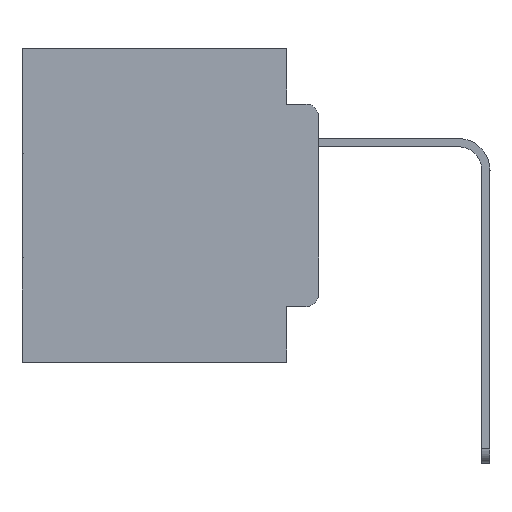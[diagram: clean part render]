
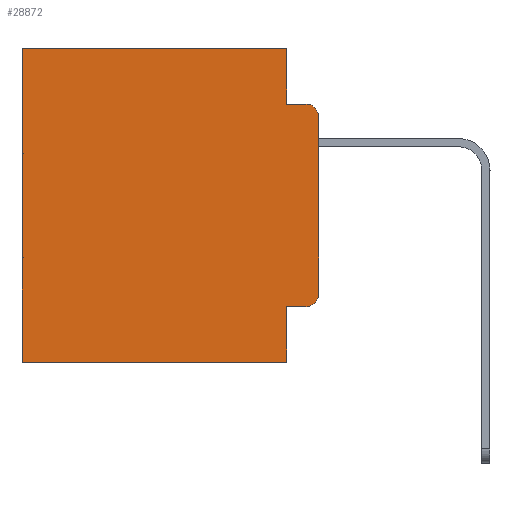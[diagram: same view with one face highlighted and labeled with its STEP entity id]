
A CAD part, left-side view. The second image highlights one B-rep face of the part: STEP entity #28872.
In plain terms, the highlighted planar face has unit normal (-1, 0, 0).
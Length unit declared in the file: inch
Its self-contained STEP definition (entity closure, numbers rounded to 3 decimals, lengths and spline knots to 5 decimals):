
#457 = AXIS2_PLACEMENT_3D ( 'NONE', #6395, #11030, #6303 ) ;
#1258 = VECTOR ( 'NONE', #29152, 39.37008 ) ;
#1271 = VERTEX_POINT ( 'NONE', #6291 ) ;
#1674 = LINE ( 'NONE', #18268, #20343 ) ;
#1702 = LINE ( 'NONE', #28573, #14700 ) ;
#1807 = EDGE_CURVE ( 'NONE', #15006, #8651, #1702, .T. ) ;
#2079 = EDGE_CURVE ( 'NONE', #19711, #15006, #1674, .T. ) ;
#3271 = VECTOR ( 'NONE', #3747, 39.37008 ) ;
#3747 = DIRECTION ( 'NONE',  ( 0., 1., 0. ) ) ;
#3829 = DIRECTION ( 'NONE',  ( 0., 0., -1. ) ) ;
#3906 = CARTESIAN_POINT ( 'NONE',  ( 0.298, 0.473, -0.5 ) ) ;
#4085 = VECTOR ( 'NONE', #28516, 39.37008 ) ;
#4306 = EDGE_CURVE ( 'NONE', #5901, #17204, #14968, .T. ) ;
#4488 = ORIENTED_EDGE ( 'NONE', *, *, #25899, .T. ) ;
#5901 = VERTEX_POINT ( 'NONE', #8008 ) ;
#6069 = EDGE_CURVE ( 'NONE', #5901, #1271, #21643, .T. ) ;
#6136 = DIRECTION ( 'NONE',  ( -1., 0., 0. ) ) ;
#6291 = CARTESIAN_POINT ( 'NONE',  ( 0.298, 0.02, -0.4115 ) ) ;
#6303 = DIRECTION ( 'NONE',  ( 0., 0., -1. ) ) ;
#6395 = CARTESIAN_POINT ( 'NONE',  ( 0.298, 0., 0. ) ) ;
#6492 = CARTESIAN_POINT ( 'NONE',  ( 0.298, 0.051, -0.5 ) ) ;
#7212 = DIRECTION ( 'NONE',  ( 0., 1., 0. ) ) ;
#7290 = EDGE_CURVE ( 'NONE', #19711, #14281, #18712, .T. ) ;
#7465 = FACE_OUTER_BOUND ( 'NONE', #13485, .T. ) ;
#7479 = VERTEX_POINT ( 'NONE', #15176 ) ;
#7544 = VECTOR ( 'NONE', #13994, 39.37008 ) ;
#8008 = CARTESIAN_POINT ( 'NONE',  ( 0.298, 0.051, -0.4115 ) ) ;
#8141 = CARTESIAN_POINT ( 'NONE',  ( 0.298, 0.051, -0.0885 ) ) ;
#8651 = VERTEX_POINT ( 'NONE', #3906 ) ;
#9332 = CARTESIAN_POINT ( 'NONE',  ( 0.298, 0.051, 0. ) ) ;
#9421 = ORIENTED_EDGE ( 'NONE', *, *, #1807, .T. ) ;
#9617 = CARTESIAN_POINT ( 'NONE',  ( 0.298, 0., -0.3915 ) ) ;
#10223 = ORIENTED_EDGE ( 'NONE', *, *, #26518, .T. ) ;
#10606 = AXIS2_PLACEMENT_3D ( 'NONE', #17167, #6136, #21711 ) ;
#10766 = DIRECTION ( 'NONE',  ( 0., 0., -1. ) ) ;
#11030 = DIRECTION ( 'NONE',  ( 1., 0., 0. ) ) ;
#11099 = CARTESIAN_POINT ( 'NONE',  ( 0.298, 0.051, 0. ) ) ;
#11452 = CARTESIAN_POINT ( 'NONE',  ( 0.298, 0.02, -0.3915 ) ) ;
#12358 = EDGE_CURVE ( 'NONE', #14281, #7479, #16742, .T. ) ;
#13448 = CARTESIAN_POINT ( 'NONE',  ( 0.298, 0., -0.1085 ) ) ;
#13485 = EDGE_LOOP ( 'NONE', ( #16006, #4488, #19543, #16410, #28604, #9421, #14288, #26752, #24125, #10223 ) ) ;
#13994 = DIRECTION ( 'NONE',  ( 0., 0., -1. ) ) ;
#14281 = VERTEX_POINT ( 'NONE', #8141 ) ;
#14288 = ORIENTED_EDGE ( 'NONE', *, *, #24759, .F. ) ;
#14700 = VECTOR ( 'NONE', #3829, 39.37008 ) ;
#14968 = LINE ( 'NONE', #9332, #1258 ) ;
#15006 = VERTEX_POINT ( 'NONE', #18141 ) ;
#15176 = CARTESIAN_POINT ( 'NONE',  ( 0.298, 0.02, -0.0885 ) ) ;
#15267 = LINE ( 'NONE', #17229, #3271 ) ;
#15993 = VERTEX_POINT ( 'NONE', #13448 ) ;
#16006 = ORIENTED_EDGE ( 'NONE', *, *, #23789, .F. ) ;
#16410 = ORIENTED_EDGE ( 'NONE', *, *, #7290, .F. ) ;
#16742 = LINE ( 'NONE', #26654, #4085 ) ;
#17167 = CARTESIAN_POINT ( 'NONE',  ( 0.298, 0.02, -0.1085 ) ) ;
#17204 = VERTEX_POINT ( 'NONE', #6492 ) ;
#17229 = CARTESIAN_POINT ( 'NONE',  ( 0.298, 0., -0.5 ) ) ;
#17386 = VECTOR ( 'NONE', #28432, 39.37008 ) ;
#17559 = CARTESIAN_POINT ( 'NONE',  ( 0.298, 0.051, -0.4115 ) ) ;
#17834 = PLANE ( 'NONE',  #457 ) ;
#18141 = CARTESIAN_POINT ( 'NONE',  ( 0.298, 0.473, 0. ) ) ;
#18262 = DIRECTION ( 'NONE',  ( -1., 0., 0. ) ) ;
#18268 = CARTESIAN_POINT ( 'NONE',  ( 0.298, 0., 0. ) ) ;
#18671 = CIRCLE ( 'NONE', #23066, 0.02 ) ;
#18712 = LINE ( 'NONE', #19744, #19419 ) ;
#19419 = VECTOR ( 'NONE', #10766, 39.37008 ) ;
#19543 = ORIENTED_EDGE ( 'NONE', *, *, #12358, .F. ) ;
#19711 = VERTEX_POINT ( 'NONE', #11099 ) ;
#19744 = CARTESIAN_POINT ( 'NONE',  ( 0.298, 0.051, 0. ) ) ;
#20266 = LINE ( 'NONE', #27530, #7544 ) ;
#20343 = VECTOR ( 'NONE', #7212, 39.37008 ) ;
#21643 = LINE ( 'NONE', #17559, #17386 ) ;
#21711 = DIRECTION ( 'NONE',  ( 0., 0., -1. ) ) ;
#23066 = AXIS2_PLACEMENT_3D ( 'NONE', #11452, #18262, #27074 ) ;
#23789 = EDGE_CURVE ( 'NONE', #15993, #27793, #20266, .T. ) ;
#24125 = ORIENTED_EDGE ( 'NONE', *, *, #6069, .T. ) ;
#24346 = CIRCLE ( 'NONE', #10606, 0.02 ) ;
#24759 = EDGE_CURVE ( 'NONE', #17204, #8651, #15267, .T. ) ;
#25899 = EDGE_CURVE ( 'NONE', #15993, #7479, #24346, .T. ) ;
#26518 = EDGE_CURVE ( 'NONE', #1271, #27793, #18671, .T. ) ;
#26654 = CARTESIAN_POINT ( 'NONE',  ( 0.298, 0.051, -0.0885 ) ) ;
#26752 = ORIENTED_EDGE ( 'NONE', *, *, #4306, .F. ) ;
#27074 = DIRECTION ( 'NONE',  ( 0., 0., -1. ) ) ;
#27530 = CARTESIAN_POINT ( 'NONE',  ( 0.298, 0., 0. ) ) ;
#27793 = VERTEX_POINT ( 'NONE', #9617 ) ;
#28432 = DIRECTION ( 'NONE',  ( 0., -1., 0. ) ) ;
#28516 = DIRECTION ( 'NONE',  ( 0., -1., 0. ) ) ;
#28573 = CARTESIAN_POINT ( 'NONE',  ( 0.298, 0.473, 0. ) ) ;
#28604 = ORIENTED_EDGE ( 'NONE', *, *, #2079, .T. ) ;
#28872 = ADVANCED_FACE ( 'NONE', ( #7465 ), #17834, .F. ) ;
#29152 = DIRECTION ( 'NONE',  ( 0., 0., -1. ) ) ;
